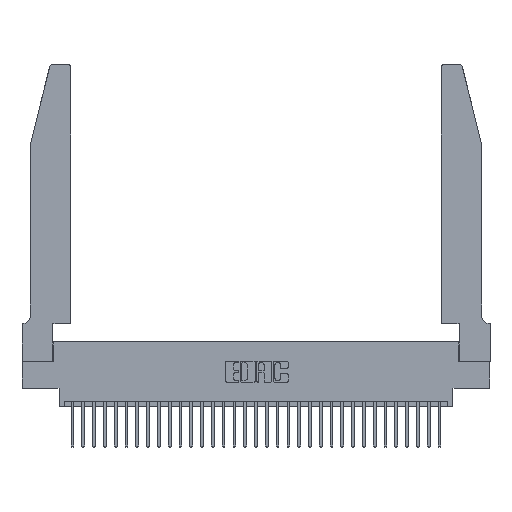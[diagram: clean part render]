
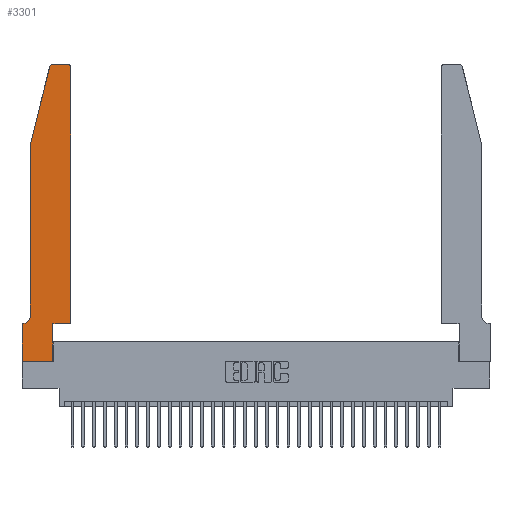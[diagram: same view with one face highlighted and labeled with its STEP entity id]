
A CAD part, top view. The second image highlights one B-rep face of the part: STEP entity #3301.
In plain terms, the highlighted planar face has unit normal (0, 0, 1).
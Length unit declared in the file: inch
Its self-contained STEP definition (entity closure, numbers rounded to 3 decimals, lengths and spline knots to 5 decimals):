
#288 = VECTOR ( 'NONE', #32801, 39.37008 ) ;
#494 = EDGE_CURVE ( 'NONE', #17668, #24761, #3444, .T. ) ;
#705 = EDGE_CURVE ( 'NONE', #746, #3609, #29205, .T. ) ;
#746 = VERTEX_POINT ( 'NONE', #11709 ) ;
#1085 = CARTESIAN_POINT ( 'NONE',  ( 0.4505, 2.72, 0.37 ) ) ;
#1293 = LINE ( 'NONE', #13613, #20232 ) ;
#1330 = EDGE_CURVE ( 'NONE', #12481, #17910, #17895, .T. ) ;
#2136 = EDGE_CURVE ( 'NONE', #29538, #24093, #15912, .T. ) ;
#2153 = ORIENTED_EDGE ( 'NONE', *, *, #6568, .T. ) ;
#2375 = CARTESIAN_POINT ( 'NONE',  ( 0.2865, 0.35, 0.37 ) ) ;
#3092 = EDGE_CURVE ( 'NONE', #17653, #17668, #28307, .T. ) ;
#3254 = CARTESIAN_POINT ( 'NONE',  ( 0.2865, 0.35, 0.37 ) ) ;
#3301 = ADVANCED_FACE ( 'NONE', ( #30711 ), #5956, .T. ) ;
#3359 = DIRECTION ( 'NONE',  ( -1., 0., 0. ) ) ;
#3444 = CIRCLE ( 'NONE', #21852, 0.03 ) ;
#3516 = DIRECTION ( 'NONE',  ( 0., 0., 1. ) ) ;
#3609 = VERTEX_POINT ( 'NONE', #2375 ) ;
#3989 = CARTESIAN_POINT ( 'NONE',  ( 0.0755, 2., 0.37 ) ) ;
#4092 = CARTESIAN_POINT ( 'NONE',  ( 0.0055, 0.42, 0.37 ) ) ;
#4831 = VERTEX_POINT ( 'NONE', #20665 ) ;
#5186 = DIRECTION ( 'NONE',  ( 0., 0., 1. ) ) ;
#5406 = CARTESIAN_POINT ( 'NONE',  ( 0.284, 2.75, 0.37 ) ) ;
#5956 = PLANE ( 'NONE',  #26424 ) ;
#6029 = EDGE_CURVE ( 'NONE', #24761, #12481, #14453, .T. ) ;
#6568 = EDGE_CURVE ( 'NONE', #28866, #746, #9890, .T. ) ;
#7039 = CARTESIAN_POINT ( 'NONE',  ( 0., 0., 0.37 ) ) ;
#7427 = VECTOR ( 'NONE', #16023, 39.37008 ) ;
#8222 = DIRECTION ( 'NONE',  ( 1., 0., 0. ) ) ;
#8331 = DIRECTION ( 'NONE',  ( 0., -1., 0. ) ) ;
#8603 = VECTOR ( 'NONE', #20357, 39.37008 ) ;
#8714 = LINE ( 'NONE', #3989, #32914 ) ;
#8763 = CARTESIAN_POINT ( 'NONE',  ( 0., 0.35, 0.37 ) ) ;
#8994 = VECTOR ( 'NONE', #3359, 39.37008 ) ;
#9278 = VERTEX_POINT ( 'NONE', #28585 ) ;
#9603 = DIRECTION ( 'NONE',  ( 1., 0., 0. ) ) ;
#9890 = LINE ( 'NONE', #7039, #19250 ) ;
#10224 = DIRECTION ( 'NONE',  ( 0., 0., 1. ) ) ;
#10653 = ORIENTED_EDGE ( 'NONE', *, *, #19117, .T. ) ;
#10924 = DIRECTION ( 'NONE',  ( 1., 0., 0. ) ) ;
#11532 = DIRECTION ( 'NONE',  ( -1., 0., 0. ) ) ;
#11709 = CARTESIAN_POINT ( 'NONE',  ( 0.2865, 0., 0.37 ) ) ;
#11915 = ORIENTED_EDGE ( 'NONE', *, *, #14151, .T. ) ;
#12209 = CARTESIAN_POINT ( 'NONE',  ( 0.2605, 2.75, 0.37 ) ) ;
#12223 = CARTESIAN_POINT ( 'NONE',  ( 0.0755, 2., 0.37 ) ) ;
#12481 = VERTEX_POINT ( 'NONE', #5406 ) ;
#13003 = CARTESIAN_POINT ( 'NONE',  ( 0.284, 2.72, 0.37 ) ) ;
#13613 = CARTESIAN_POINT ( 'NONE',  ( 0.4505, 0.35, 0.37 ) ) ;
#14151 = EDGE_CURVE ( 'NONE', #24093, #28866, #28509, .T. ) ;
#14250 = EDGE_CURVE ( 'NONE', #17910, #4831, #8714, .T. ) ;
#14453 = LINE ( 'NONE', #12209, #288 ) ;
#14691 = ORIENTED_EDGE ( 'NONE', *, *, #14250, .T. ) ;
#15231 = ORIENTED_EDGE ( 'NONE', *, *, #2136, .T. ) ;
#15391 = CARTESIAN_POINT ( 'NONE',  ( 0.4505, 0.35, 0.37 ) ) ;
#15818 = VECTOR ( 'NONE', #25830, 39.37008 ) ;
#15912 = LINE ( 'NONE', #16125, #8994 ) ;
#16023 = DIRECTION ( 'NONE',  ( 0., 1., 0. ) ) ;
#16072 = CARTESIAN_POINT ( 'NONE',  ( 0., 0., 0.37 ) ) ;
#16125 = CARTESIAN_POINT ( 'NONE',  ( 0.0755, 0.35, 0.37 ) ) ;
#17653 = VERTEX_POINT ( 'NONE', #26627 ) ;
#17668 = VERTEX_POINT ( 'NONE', #1085 ) ;
#17874 = ORIENTED_EDGE ( 'NONE', *, *, #1330, .T. ) ;
#17895 = CIRCLE ( 'NONE', #30701, 0.03 ) ;
#17910 = VERTEX_POINT ( 'NONE', #22458 ) ;
#19117 = EDGE_CURVE ( 'NONE', #4831, #9278, #19149, .T. ) ;
#19149 = LINE ( 'NONE', #12223, #8603 ) ;
#19250 = VECTOR ( 'NONE', #9603, 39.37008 ) ;
#20232 = VECTOR ( 'NONE', #29586, 39.37008 ) ;
#20340 = EDGE_LOOP ( 'NONE', ( #25663, #17874, #14691, #10653, #27263, #15231, #11915, #2153, #25611, #26268, #32646, #26327 ) ) ;
#20357 = DIRECTION ( 'NONE',  ( 0., -1., 0. ) ) ;
#20665 = CARTESIAN_POINT ( 'NONE',  ( 0.0755, 2., 0.37 ) ) ;
#21852 = AXIS2_PLACEMENT_3D ( 'NONE', #33023, #10224, #8222 ) ;
#22021 = EDGE_CURVE ( 'NONE', #9278, #29538, #33253, .T. ) ;
#22025 = DIRECTION ( 'NONE',  ( -0.239, -0.971, 0. ) ) ;
#22458 = CARTESIAN_POINT ( 'NONE',  ( 0.25487, 2.72718, 0.37 ) ) ;
#24016 = DIRECTION ( 'NONE',  ( 1., 0., 0. ) ) ;
#24093 = VERTEX_POINT ( 'NONE', #29684 ) ;
#24761 = VERTEX_POINT ( 'NONE', #25024 ) ;
#25024 = CARTESIAN_POINT ( 'NONE',  ( 0.4205, 2.75, 0.37 ) ) ;
#25611 = ORIENTED_EDGE ( 'NONE', *, *, #705, .T. ) ;
#25663 = ORIENTED_EDGE ( 'NONE', *, *, #6029, .T. ) ;
#25830 = DIRECTION ( 'NONE',  ( 0., 1., 0. ) ) ;
#26268 = ORIENTED_EDGE ( 'NONE', *, *, #30148, .T. ) ;
#26327 = ORIENTED_EDGE ( 'NONE', *, *, #494, .T. ) ;
#26424 = AXIS2_PLACEMENT_3D ( 'NONE', #8763, #3516, #24016 ) ;
#26627 = CARTESIAN_POINT ( 'NONE',  ( 0.4505, 0.35, 0.37 ) ) ;
#27084 = CARTESIAN_POINT ( 'NONE',  ( 0., 0., 0.37 ) ) ;
#27090 = DIRECTION ( 'NONE',  ( 0., 0., -1. ) ) ;
#27263 = ORIENTED_EDGE ( 'NONE', *, *, #22021, .T. ) ;
#28281 = AXIS2_PLACEMENT_3D ( 'NONE', #4092, #27090, #11532 ) ;
#28307 = LINE ( 'NONE', #15391, #15818 ) ;
#28509 = LINE ( 'NONE', #16072, #29313 ) ;
#28585 = CARTESIAN_POINT ( 'NONE',  ( 0.0755, 0.42, 0.37 ) ) ;
#28866 = VERTEX_POINT ( 'NONE', #27084 ) ;
#29205 = LINE ( 'NONE', #3254, #7427 ) ;
#29313 = VECTOR ( 'NONE', #8331, 39.37008 ) ;
#29538 = VERTEX_POINT ( 'NONE', #29735 ) ;
#29586 = DIRECTION ( 'NONE',  ( 1., 0., 0. ) ) ;
#29684 = CARTESIAN_POINT ( 'NONE',  ( 0., 0.35, 0.37 ) ) ;
#29735 = CARTESIAN_POINT ( 'NONE',  ( 0.0055, 0.35, 0.37 ) ) ;
#30148 = EDGE_CURVE ( 'NONE', #3609, #17653, #1293, .T. ) ;
#30701 = AXIS2_PLACEMENT_3D ( 'NONE', #13003, #5186, #10924 ) ;
#30711 = FACE_OUTER_BOUND ( 'NONE', #20340, .T. ) ;
#32646 = ORIENTED_EDGE ( 'NONE', *, *, #3092, .T. ) ;
#32801 = DIRECTION ( 'NONE',  ( -1., 0., 0. ) ) ;
#32914 = VECTOR ( 'NONE', #22025, 39.37008 ) ;
#33023 = CARTESIAN_POINT ( 'NONE',  ( 0.4205, 2.72, 0.37 ) ) ;
#33253 = CIRCLE ( 'NONE', #28281, 0.07 ) ;
